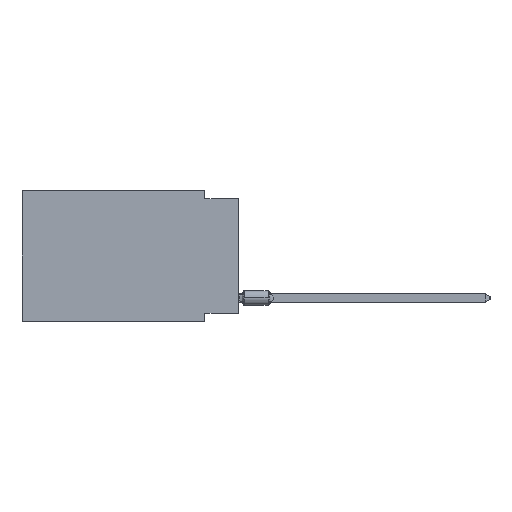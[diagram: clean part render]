
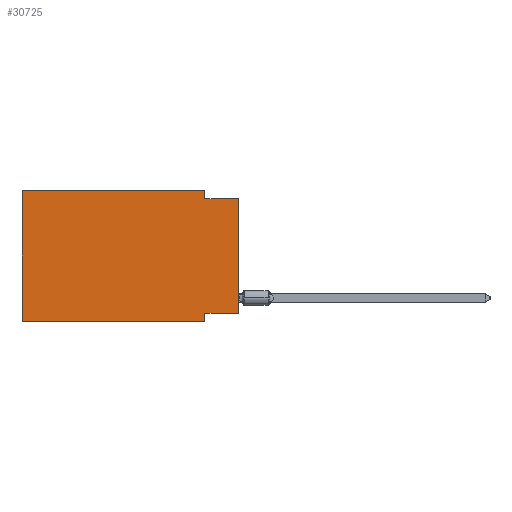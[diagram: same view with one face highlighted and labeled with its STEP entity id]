
A CAD part, left-side view. The second image highlights one B-rep face of the part: STEP entity #30725.
In plain terms, the highlighted planar face has unit normal (-1, 0, 0).
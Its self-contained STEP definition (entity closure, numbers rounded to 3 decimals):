
#98 = DIRECTION ( 'NONE',  ( 1., 0., 0. ) ) ;
#412 = ORIENTED_EDGE ( 'NONE', *, *, #746, .F. ) ;
#746 = EDGE_CURVE ( 'NONE', #57971, #53842, #41767, .T. ) ;
#899 = VECTOR ( 'NONE', #19689, 1000. ) ;
#932 = ORIENTED_EDGE ( 'NONE', *, *, #2770, .F. ) ;
#1147 = EDGE_CURVE ( 'NONE', #10394, #30269, #14725, .T. ) ;
#1592 = CARTESIAN_POINT ( 'NONE',  ( 0., 0., -9.271 ) ) ;
#2770 = EDGE_CURVE ( 'NONE', #15287, #8940, #6125, .T. ) ;
#4700 = LINE ( 'NONE', #48963, #40699 ) ;
#5084 = CARTESIAN_POINT ( 'NONE',  ( 0., 16.383, 0. ) ) ;
#6125 = LINE ( 'NONE', #28699, #43931 ) ;
#7950 = EDGE_CURVE ( 'NONE', #57971, #49441, #41957, .T. ) ;
#8897 = DIRECTION ( 'NONE',  ( 0., 0., -1. ) ) ;
#8940 = VERTEX_POINT ( 'NONE', #39733 ) ;
#9936 = CARTESIAN_POINT ( 'NONE',  ( 0., 16.383, -9.906 ) ) ;
#10219 = AXIS2_PLACEMENT_3D ( 'NONE', #5084, #98, #8897 ) ;
#10394 = VERTEX_POINT ( 'NONE', #9936 ) ;
#11463 = CARTESIAN_POINT ( 'NONE',  ( 0., 0., 0. ) ) ;
#11718 = CARTESIAN_POINT ( 'NONE',  ( 0., 2.54, -9.906 ) ) ;
#11792 = EDGE_CURVE ( 'NONE', #53842, #28938, #4700, .T. ) ;
#14151 = CARTESIAN_POINT ( 'NONE',  ( 0., 16.383, 0. ) ) ;
#14725 = LINE ( 'NONE', #14151, #899 ) ;
#15287 = VERTEX_POINT ( 'NONE', #44248 ) ;
#17121 = DIRECTION ( 'NONE',  ( 0., -1., 0. ) ) ;
#17125 = FACE_OUTER_BOUND ( 'NONE', #51209, .T. ) ;
#17189 = ORIENTED_EDGE ( 'NONE', *, *, #11792, .F. ) ;
#17987 = VECTOR ( 'NONE', #53958, 1000. ) ;
#18175 = LINE ( 'NONE', #44877, #17987 ) ;
#18258 = CARTESIAN_POINT ( 'NONE',  ( 0., 16.383, -9.906 ) ) ;
#18674 = VECTOR ( 'NONE', #17121, 1000. ) ;
#19556 = VECTOR ( 'NONE', #46746, 1000. ) ;
#19689 = DIRECTION ( 'NONE',  ( 0., 0., 1. ) ) ;
#20309 = VECTOR ( 'NONE', #42576, 1000. ) ;
#23716 = CARTESIAN_POINT ( 'NONE',  ( 0., 2.54, -9.271 ) ) ;
#24804 = ORIENTED_EDGE ( 'NONE', *, *, #39739, .F. ) ;
#27069 = LINE ( 'NONE', #18258, #18674 ) ;
#28580 = CARTESIAN_POINT ( 'NONE',  ( 0., 0., -9.271 ) ) ;
#28699 = CARTESIAN_POINT ( 'NONE',  ( 0., 2.54, 0. ) ) ;
#28938 = VERTEX_POINT ( 'NONE', #11718 ) ;
#29352 = DIRECTION ( 'NONE',  ( 0., 0., 1. ) ) ;
#29418 = VECTOR ( 'NONE', #29352, 1000. ) ;
#29490 = EDGE_CURVE ( 'NONE', #10394, #28938, #27069, .T. ) ;
#30269 = VERTEX_POINT ( 'NONE', #42218 ) ;
#30725 = ADVANCED_FACE ( 'NONE', ( #17125 ), #49065, .F. ) ;
#31880 = ORIENTED_EDGE ( 'NONE', *, *, #29490, .T. ) ;
#33911 = ORIENTED_EDGE ( 'NONE', *, *, #1147, .F. ) ;
#34325 = EDGE_CURVE ( 'NONE', #8940, #49441, #18175, .T. ) ;
#35834 = ORIENTED_EDGE ( 'NONE', *, *, #7950, .T. ) ;
#38378 = DIRECTION ( 'NONE',  ( 0., 0., -1. ) ) ;
#38768 = CARTESIAN_POINT ( 'NONE',  ( 0., 16.383, 0. ) ) ;
#39733 = CARTESIAN_POINT ( 'NONE',  ( 0., 2.54, -0.635 ) ) ;
#39739 = EDGE_CURVE ( 'NONE', #30269, #15287, #47262, .T. ) ;
#40699 = VECTOR ( 'NONE', #53657, 1000. ) ;
#41767 = LINE ( 'NONE', #1592, #19556 ) ;
#41957 = LINE ( 'NONE', #11463, #29418 ) ;
#42218 = CARTESIAN_POINT ( 'NONE',  ( 0., 16.383, 0. ) ) ;
#42576 = DIRECTION ( 'NONE',  ( 0., -1., 0. ) ) ;
#43931 = VECTOR ( 'NONE', #38378, 1000. ) ;
#44248 = CARTESIAN_POINT ( 'NONE',  ( 0., 2.54, 0. ) ) ;
#44877 = CARTESIAN_POINT ( 'NONE',  ( 0., 0., -0.635 ) ) ;
#46746 = DIRECTION ( 'NONE',  ( 0., 1., 0. ) ) ;
#47262 = LINE ( 'NONE', #38768, #20309 ) ;
#48963 = CARTESIAN_POINT ( 'NONE',  ( 0., 2.54, -9.906 ) ) ;
#49065 = PLANE ( 'NONE',  #10219 ) ;
#49441 = VERTEX_POINT ( 'NONE', #57013 ) ;
#51209 = EDGE_LOOP ( 'NONE', ( #35834, #56417, #932, #24804, #33911, #31880, #17189, #412 ) ) ;
#53657 = DIRECTION ( 'NONE',  ( 0., 0., -1. ) ) ;
#53842 = VERTEX_POINT ( 'NONE', #23716 ) ;
#53958 = DIRECTION ( 'NONE',  ( 0., -1., 0. ) ) ;
#56417 = ORIENTED_EDGE ( 'NONE', *, *, #34325, .F. ) ;
#57013 = CARTESIAN_POINT ( 'NONE',  ( 0., 0., -0.635 ) ) ;
#57971 = VERTEX_POINT ( 'NONE', #28580 ) ;
